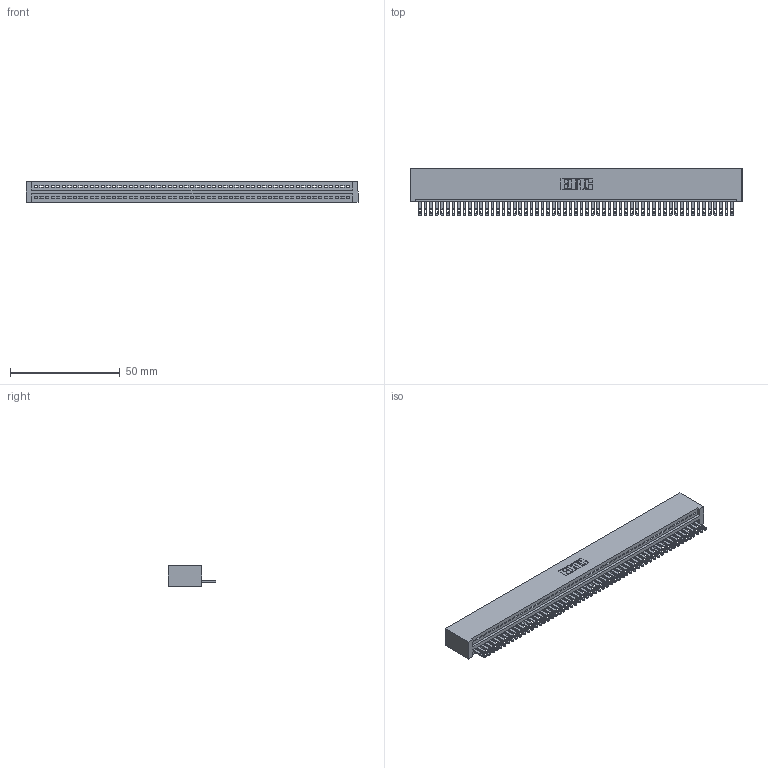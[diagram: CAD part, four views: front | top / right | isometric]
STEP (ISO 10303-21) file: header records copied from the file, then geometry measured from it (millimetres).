
FILE_DESCRIPTION (( 'STEP AP203' ), '1' );
FILE_NAME ('895-057-500-101.STEP', '2020-09-27T17:04:58', ( '' ), ( '' ), 'SwSTEP 2.0', 'SolidWorks 2020', '' );
FILE_SCHEMA (( 'CONFIG_CONTROL_DESIGN' ));
Length unit declared in the file: inch
Products named in the file (3): 345-292-001_345-293-100; 895-057-500-101; 845 Part_No Mounting Lugs
Assembly tree (58 placements, depth 2):
  895-057-500-101
    845 Part_No Mounting Lugs
    345-292-001_345-293-100  x57
Bounding box: 151.38 x 21.51 x 9.4 mm (x, y, z)
Volume: 15121.1 mm3; surface area: 20616.6 mm2
Topology: 58 solids, 58 shells, 3196 faces, 9893 edges, 6594 vertices
Faces by surface type: plane 2014, cylinder 1182
Entity records: 40533 total; most frequent: CARTESIAN_POINT 7027, ORIENTED_EDGE 7018, DIRECTION 6111, EDGE_CURVE 3509, VECTOR 3153, LINE 3153, VERTEX_POINT 2338, AXIS2_PLACEMENT_3D 1479
